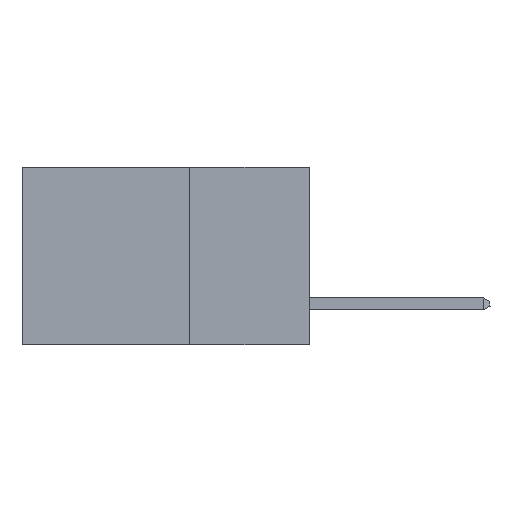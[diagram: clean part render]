
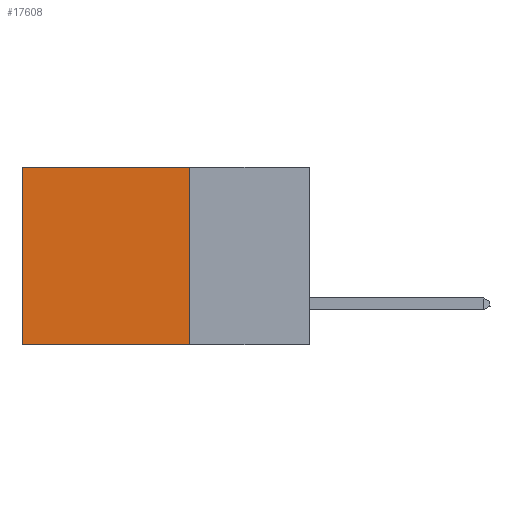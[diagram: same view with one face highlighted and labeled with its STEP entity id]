
A CAD part, left-side view. The second image highlights one B-rep face of the part: STEP entity #17608.
In plain terms, the highlighted planar face has unit normal (-1, 0, 0).
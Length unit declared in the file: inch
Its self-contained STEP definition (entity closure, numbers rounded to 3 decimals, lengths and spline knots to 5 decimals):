
#204 = LINE ( 'NONE', #7881, #17777 ) ;
#625 = CARTESIAN_POINT ( 'NONE',  ( 0.2875, 0.6, 0. ) ) ;
#876 = CARTESIAN_POINT ( 'NONE',  ( 0.2875, 0.25, 0. ) ) ;
#2150 = VERTEX_POINT ( 'NONE', #5553 ) ;
#2602 = EDGE_CURVE ( 'NONE', #8913, #2150, #204, .T. ) ;
#2852 = VERTEX_POINT ( 'NONE', #7044 ) ;
#3135 = LINE ( 'NONE', #15244, #17334 ) ;
#3213 = CARTESIAN_POINT ( 'NONE',  ( 0.2875, 0.25, -0.37 ) ) ;
#3803 = DIRECTION ( 'NONE',  ( 0., 1., 0. ) ) ;
#4588 = VECTOR ( 'NONE', #3803, 39.37008 ) ;
#4657 = ORIENTED_EDGE ( 'NONE', *, *, #4665, .T. ) ;
#4665 = EDGE_CURVE ( 'NONE', #2852, #11254, #8678, .T. ) ;
#4804 = EDGE_LOOP ( 'NONE', ( #8504, #17911, #8790, #4657 ) ) ;
#5553 = CARTESIAN_POINT ( 'NONE',  ( 0.2875, 0.6, -0.37 ) ) ;
#5701 = CARTESIAN_POINT ( 'NONE',  ( 0.2875, 0.6, 0. ) ) ;
#6200 = DIRECTION ( 'NONE',  ( 1., 0., 0. ) ) ;
#6578 = EDGE_CURVE ( 'NONE', #11254, #2150, #14780, .T. ) ;
#7044 = CARTESIAN_POINT ( 'NONE',  ( 0.2875, 0.25, 0. ) ) ;
#7462 = EDGE_CURVE ( 'NONE', #2852, #8913, #3135, .T. ) ;
#7881 = CARTESIAN_POINT ( 'NONE',  ( 0.2875, 0.25, -0.37 ) ) ;
#8504 = ORIENTED_EDGE ( 'NONE', *, *, #6578, .T. ) ;
#8678 = LINE ( 'NONE', #876, #4588 ) ;
#8790 = ORIENTED_EDGE ( 'NONE', *, *, #7462, .F. ) ;
#8913 = VERTEX_POINT ( 'NONE', #3213 ) ;
#9056 = DIRECTION ( 'NONE',  ( 0., 0., -1. ) ) ;
#9315 = AXIS2_PLACEMENT_3D ( 'NONE', #11618, #6200, #15727 ) ;
#11146 = VECTOR ( 'NONE', #9056, 39.37008 ) ;
#11254 = VERTEX_POINT ( 'NONE', #5701 ) ;
#11618 = CARTESIAN_POINT ( 'NONE',  ( 0.2875, 0.25, 0. ) ) ;
#11698 = FACE_OUTER_BOUND ( 'NONE', #4804, .T. ) ;
#14780 = LINE ( 'NONE', #625, #11146 ) ;
#15244 = CARTESIAN_POINT ( 'NONE',  ( 0.2875, 0.25, 0. ) ) ;
#15672 = PLANE ( 'NONE',  #9315 ) ;
#15727 = DIRECTION ( 'NONE',  ( 0., 0., -1. ) ) ;
#16032 = DIRECTION ( 'NONE',  ( 0., 1., 0. ) ) ;
#16610 = DIRECTION ( 'NONE',  ( 0., 0., -1. ) ) ;
#17334 = VECTOR ( 'NONE', #16610, 39.37008 ) ;
#17608 = ADVANCED_FACE ( 'NONE', ( #11698 ), #15672, .F. ) ;
#17777 = VECTOR ( 'NONE', #16032, 39.37008 ) ;
#17911 = ORIENTED_EDGE ( 'NONE', *, *, #2602, .F. ) ;
